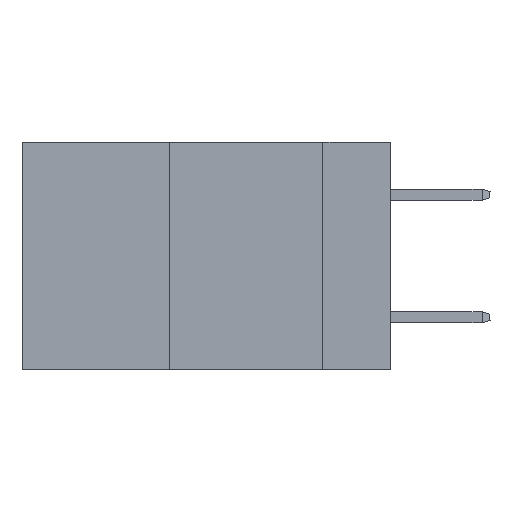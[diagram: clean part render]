
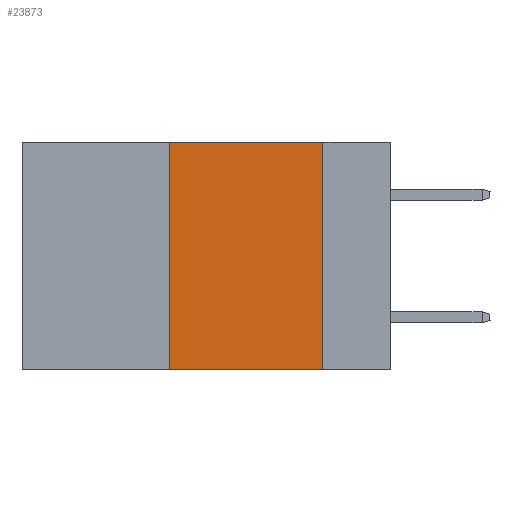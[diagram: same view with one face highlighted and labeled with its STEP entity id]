
A CAD part, left-side view. The second image highlights one B-rep face of the part: STEP entity #23873.
In plain terms, the highlighted planar face has unit normal (-1, 0, 0).
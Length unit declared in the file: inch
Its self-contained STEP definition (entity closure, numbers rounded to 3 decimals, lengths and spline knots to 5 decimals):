
#197 = VECTOR ( 'NONE', #4051, 39.37008 ) ;
#566 = DIRECTION ( 'NONE',  ( 0., -1., 0. ) ) ;
#2491 = FACE_OUTER_BOUND ( 'NONE', #17206, .T. ) ;
#2723 = DIRECTION ( 'NONE',  ( 0., 0., -1. ) ) ;
#3404 = ORIENTED_EDGE ( 'NONE', *, *, #17916, .F. ) ;
#4051 = DIRECTION ( 'NONE',  ( 0., 0., 1. ) ) ;
#4445 = EDGE_CURVE ( 'NONE', #47073, #40185, #26609, .T. ) ;
#4585 = ORIENTED_EDGE ( 'NONE', *, *, #35256, .F. ) ;
#6251 = ORIENTED_EDGE ( 'NONE', *, *, #4445, .F. ) ;
#7479 = CARTESIAN_POINT ( 'NONE',  ( 0., 0.6, -0.37 ) ) ;
#7524 = AXIS2_PLACEMENT_3D ( 'NONE', #39621, #46645, #2723 ) ;
#8145 = CARTESIAN_POINT ( 'NONE',  ( 0., 0.11, 0. ) ) ;
#8736 = CARTESIAN_POINT ( 'NONE',  ( 0., 0.36, -0.37 ) ) ;
#11136 = DIRECTION ( 'NONE',  ( 0., -1., 0. ) ) ;
#12041 = ORIENTED_EDGE ( 'NONE', *, *, #15325, .T. ) ;
#12471 = VERTEX_POINT ( 'NONE', #40740 ) ;
#15325 = EDGE_CURVE ( 'NONE', #31855, #12471, #41741, .T. ) ;
#16947 = CARTESIAN_POINT ( 'NONE',  ( 0., 0.36, 0. ) ) ;
#17206 = EDGE_LOOP ( 'NONE', ( #4585, #6251, #3404, #12041 ) ) ;
#17916 = EDGE_CURVE ( 'NONE', #31855, #47073, #45528, .T. ) ;
#19167 = DIRECTION ( 'NONE',  ( 0., 0., -1. ) ) ;
#20771 = PLANE ( 'NONE',  #7524 ) ;
#23873 = ADVANCED_FACE ( 'NONE', ( #2491 ), #20771, .F. ) ;
#24314 = VECTOR ( 'NONE', #566, 39.37008 ) ;
#26609 = LINE ( 'NONE', #33603, #24314 ) ;
#27332 = VECTOR ( 'NONE', #11136, 39.37008 ) ;
#30314 = CARTESIAN_POINT ( 'NONE',  ( 0., 0.36, 0. ) ) ;
#31855 = VERTEX_POINT ( 'NONE', #8736 ) ;
#33603 = CARTESIAN_POINT ( 'NONE',  ( 0., 0.6, 0. ) ) ;
#33697 = LINE ( 'NONE', #8145, #45770 ) ;
#34085 = CARTESIAN_POINT ( 'NONE',  ( 0., 0.11, 0. ) ) ;
#35256 = EDGE_CURVE ( 'NONE', #40185, #12471, #33697, .T. ) ;
#39621 = CARTESIAN_POINT ( 'NONE',  ( 0., 0.6, 0. ) ) ;
#40185 = VERTEX_POINT ( 'NONE', #34085 ) ;
#40740 = CARTESIAN_POINT ( 'NONE',  ( 0., 0.11, -0.37 ) ) ;
#41741 = LINE ( 'NONE', #7479, #27332 ) ;
#45528 = LINE ( 'NONE', #30314, #197 ) ;
#45770 = VECTOR ( 'NONE', #19167, 39.37008 ) ;
#46645 = DIRECTION ( 'NONE',  ( 1., 0., 0. ) ) ;
#47073 = VERTEX_POINT ( 'NONE', #16947 ) ;
